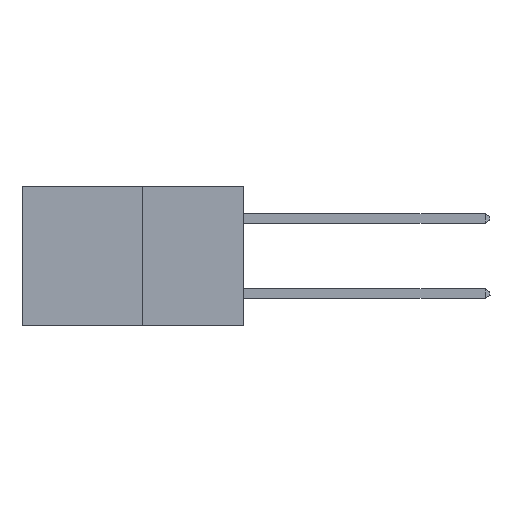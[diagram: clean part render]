
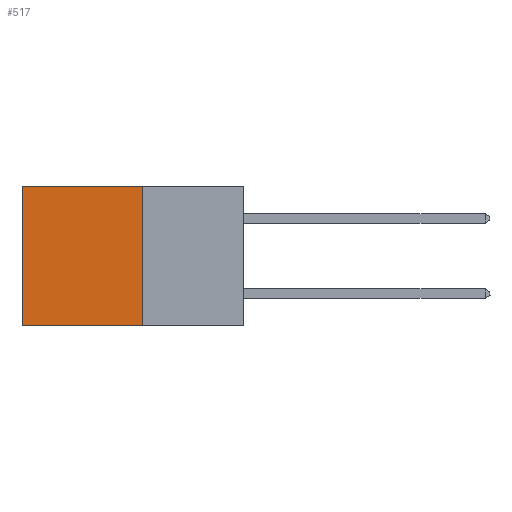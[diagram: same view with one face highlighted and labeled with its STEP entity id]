
A CAD part, left-side view. The second image highlights one B-rep face of the part: STEP entity #517.
In plain terms, the highlighted planar face has unit normal (-1, 0, 0).
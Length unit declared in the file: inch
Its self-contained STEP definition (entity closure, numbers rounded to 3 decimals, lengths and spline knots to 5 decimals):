
#177 = VECTOR ( 'NONE', #9271, 39.37008 ) ;
#261 = EDGE_LOOP ( 'NONE', ( #1849, #5680, #4278, #10043 ) ) ;
#393 = LINE ( 'NONE', #10240, #2597 ) ;
#410 = CARTESIAN_POINT ( 'NONE',  ( 0.277, 0.27, 0. ) ) ;
#488 = PLANE ( 'NONE',  #9360 ) ;
#517 = ADVANCED_FACE ( 'NONE', ( #4734 ), #488, .F. ) ;
#1575 = DIRECTION ( 'NONE',  ( 0., 0., -1. ) ) ;
#1849 = ORIENTED_EDGE ( 'NONE', *, *, #7305, .T. ) ;
#1888 = VERTEX_POINT ( 'NONE', #410 ) ;
#1977 = LINE ( 'NONE', #7339, #6137 ) ;
#2496 = CARTESIAN_POINT ( 'NONE',  ( 0.277, 0.27, -0.37 ) ) ;
#2597 = VECTOR ( 'NONE', #1575, 39.37008 ) ;
#3486 = DIRECTION ( 'NONE',  ( 0., 0., -1. ) ) ;
#3508 = CARTESIAN_POINT ( 'NONE',  ( 0.277, 0.27, -0.37 ) ) ;
#3716 = EDGE_CURVE ( 'NONE', #7819, #4077, #1977, .T. ) ;
#3799 = DIRECTION ( 'NONE',  ( 0., 1., 0. ) ) ;
#4077 = VERTEX_POINT ( 'NONE', #7999 ) ;
#4186 = VERTEX_POINT ( 'NONE', #7806 ) ;
#4278 = ORIENTED_EDGE ( 'NONE', *, *, #5233, .F. ) ;
#4687 = LINE ( 'NONE', #10041, #177 ) ;
#4734 = FACE_OUTER_BOUND ( 'NONE', #261, .T. ) ;
#5103 = LINE ( 'NONE', #5149, #8908 ) ;
#5149 = CARTESIAN_POINT ( 'NONE',  ( 0.277, 0.59, -0.37 ) ) ;
#5233 = EDGE_CURVE ( 'NONE', #1888, #7819, #393, .T. ) ;
#5557 = DIRECTION ( 'NONE',  ( 1., 0., 0. ) ) ;
#5680 = ORIENTED_EDGE ( 'NONE', *, *, #3716, .F. ) ;
#6137 = VECTOR ( 'NONE', #3799, 39.37008 ) ;
#7305 = EDGE_CURVE ( 'NONE', #4186, #4077, #5103, .T. ) ;
#7339 = CARTESIAN_POINT ( 'NONE',  ( 0.277, 0.27, -0.37 ) ) ;
#7806 = CARTESIAN_POINT ( 'NONE',  ( 0.277, 0.59, 0. ) ) ;
#7819 = VERTEX_POINT ( 'NONE', #2496 ) ;
#7999 = CARTESIAN_POINT ( 'NONE',  ( 0.277, 0.59, -0.37 ) ) ;
#8562 = DIRECTION ( 'NONE',  ( 0., 0., -1. ) ) ;
#8908 = VECTOR ( 'NONE', #8562, 39.37008 ) ;
#9146 = EDGE_CURVE ( 'NONE', #1888, #4186, #4687, .T. ) ;
#9271 = DIRECTION ( 'NONE',  ( 0., 1., 0. ) ) ;
#9360 = AXIS2_PLACEMENT_3D ( 'NONE', #3508, #5557, #3486 ) ;
#10041 = CARTESIAN_POINT ( 'NONE',  ( 0.277, 0.27, 0. ) ) ;
#10043 = ORIENTED_EDGE ( 'NONE', *, *, #9146, .T. ) ;
#10240 = CARTESIAN_POINT ( 'NONE',  ( 0.277, 0.27, -0.37 ) ) ;
